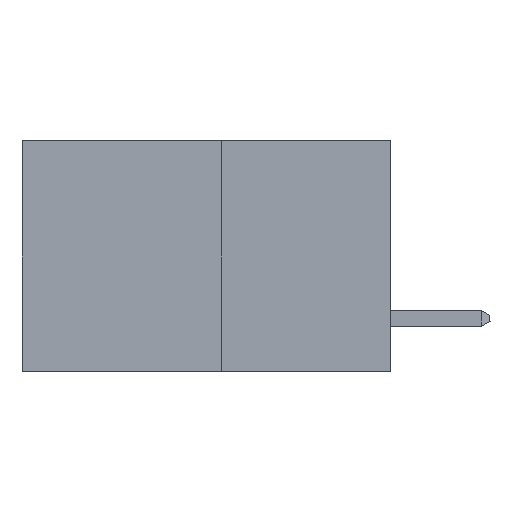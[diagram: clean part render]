
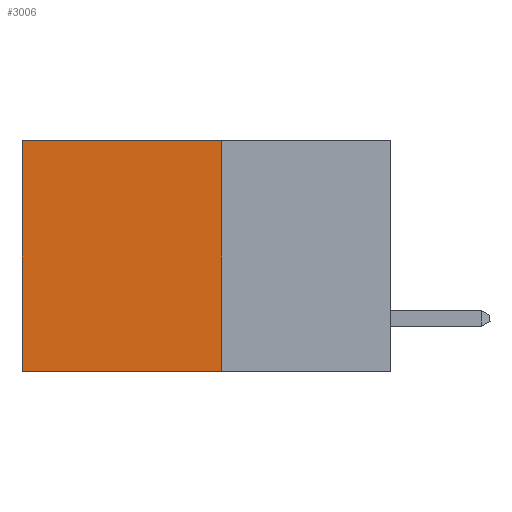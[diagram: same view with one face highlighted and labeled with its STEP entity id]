
A CAD part, left-side view. The second image highlights one B-rep face of the part: STEP entity #3006.
In plain terms, the highlighted planar face has unit normal (-1, 0, 0).
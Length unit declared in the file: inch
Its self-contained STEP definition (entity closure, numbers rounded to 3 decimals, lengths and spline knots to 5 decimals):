
#422 = EDGE_LOOP ( 'NONE', ( #4160, #882, #9007, #9842 ) ) ;
#615 = CARTESIAN_POINT ( 'NONE',  ( 0.277, 0.59, -0.37 ) ) ;
#675 = CARTESIAN_POINT ( 'NONE',  ( 0.277, 0.59, 0. ) ) ;
#698 = EDGE_CURVE ( 'NONE', #8708, #3815, #9662, .T. ) ;
#882 = ORIENTED_EDGE ( 'NONE', *, *, #6069, .F. ) ;
#1206 = DIRECTION ( 'NONE',  ( 0., 0., -1. ) ) ;
#1473 = PLANE ( 'NONE',  #10695 ) ;
#1856 = CARTESIAN_POINT ( 'NONE',  ( 0.277, 0.27, -0.37 ) ) ;
#2107 = LINE ( 'NONE', #2251, #6881 ) ;
#2201 = DIRECTION ( 'NONE',  ( 0., 1., 0. ) ) ;
#2251 = CARTESIAN_POINT ( 'NONE',  ( 0.277, 0.27, 0. ) ) ;
#2594 = CARTESIAN_POINT ( 'NONE',  ( 0.277, 0.59, -0.37 ) ) ;
#2987 = DIRECTION ( 'NONE',  ( 0., 0., -1. ) ) ;
#3006 = ADVANCED_FACE ( 'NONE', ( #5979 ), #1473, .F. ) ;
#3110 = VERTEX_POINT ( 'NONE', #1856 ) ;
#3122 = LINE ( 'NONE', #7844, #7566 ) ;
#3332 = VECTOR ( 'NONE', #7895, 39.37008 ) ;
#3637 = CARTESIAN_POINT ( 'NONE',  ( 0.277, 0.27, 0. ) ) ;
#3815 = VERTEX_POINT ( 'NONE', #615 ) ;
#4160 = ORIENTED_EDGE ( 'NONE', *, *, #698, .T. ) ;
#4424 = VECTOR ( 'NONE', #2987, 39.37008 ) ;
#5028 = VERTEX_POINT ( 'NONE', #3637 ) ;
#5979 = FACE_OUTER_BOUND ( 'NONE', #422, .T. ) ;
#6069 = EDGE_CURVE ( 'NONE', #3110, #3815, #7768, .T. ) ;
#6422 = DIRECTION ( 'NONE',  ( 0., 0., -1. ) ) ;
#6549 = EDGE_CURVE ( 'NONE', #5028, #8708, #2107, .T. ) ;
#6821 = DIRECTION ( 'NONE',  ( 1., 0., 0. ) ) ;
#6853 = CARTESIAN_POINT ( 'NONE',  ( 0.277, 0.27, -0.37 ) ) ;
#6881 = VECTOR ( 'NONE', #2201, 39.37008 ) ;
#7566 = VECTOR ( 'NONE', #1206, 39.37008 ) ;
#7768 = LINE ( 'NONE', #8011, #3332 ) ;
#7844 = CARTESIAN_POINT ( 'NONE',  ( 0.277, 0.27, -0.37 ) ) ;
#7895 = DIRECTION ( 'NONE',  ( 0., 1., 0. ) ) ;
#8011 = CARTESIAN_POINT ( 'NONE',  ( 0.277, 0.27, -0.37 ) ) ;
#8708 = VERTEX_POINT ( 'NONE', #675 ) ;
#9007 = ORIENTED_EDGE ( 'NONE', *, *, #9070, .F. ) ;
#9070 = EDGE_CURVE ( 'NONE', #5028, #3110, #3122, .T. ) ;
#9662 = LINE ( 'NONE', #2594, #4424 ) ;
#9842 = ORIENTED_EDGE ( 'NONE', *, *, #6549, .T. ) ;
#10695 = AXIS2_PLACEMENT_3D ( 'NONE', #6853, #6821, #6422 ) ;
